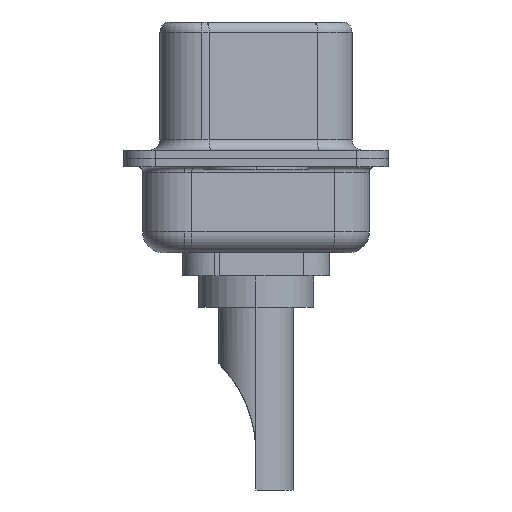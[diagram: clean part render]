
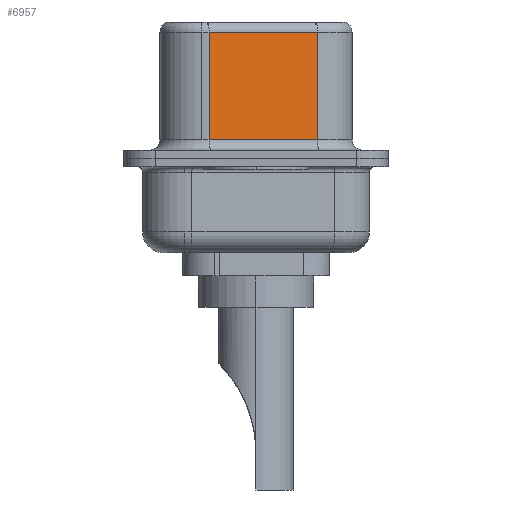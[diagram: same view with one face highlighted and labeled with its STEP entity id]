
A CAD part, left-side view. The second image highlights one B-rep face of the part: STEP entity #6957.
In plain terms, the highlighted planar face has unit normal (-0.985, -0.174, 0).
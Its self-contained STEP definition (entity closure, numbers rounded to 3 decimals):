
#53 = DIRECTION ( 'NONE',  ( -0.174, 0.985, 0. ) ) ;
#295 = ORIENTED_EDGE ( 'NONE', *, *, #6618, .T. ) ;
#870 = VECTOR ( 'NONE', #53, 1000. ) ;
#965 = EDGE_LOOP ( 'NONE', ( #12401, #5274, #295, #13449 ) ) ;
#2499 = DIRECTION ( 'NONE',  ( 0.985, 0.174, 0. ) ) ;
#2559 = CARTESIAN_POINT ( 'NONE',  ( 4.58, -2.927, 0.9 ) ) ;
#2698 = DIRECTION ( 'NONE',  ( 0.174, -0.985, 0. ) ) ;
#2806 = LINE ( 'NONE', #12154, #4554 ) ;
#3654 = LINE ( 'NONE', #13405, #870 ) ;
#4087 = AXIS2_PLACEMENT_3D ( 'NONE', #7113, #2499, #13727 ) ;
#4237 = CARTESIAN_POINT ( 'NONE',  ( 4.58, -2.927, 0.9 ) ) ;
#4554 = VECTOR ( 'NONE', #14371, 1000. ) ;
#5274 = ORIENTED_EDGE ( 'NONE', *, *, #7199, .T. ) ;
#5298 = VERTEX_POINT ( 'NONE', #12164 ) ;
#6618 = EDGE_CURVE ( 'NONE', #5298, #6783, #2806, .T. ) ;
#6783 = VERTEX_POINT ( 'NONE', #10796 ) ;
#6957 = ADVANCED_FACE ( 'NONE', ( #10961 ), #8876, .F. ) ;
#7016 = CARTESIAN_POINT ( 'NONE',  ( 4.58, -2.927, 6.52 ) ) ;
#7113 = CARTESIAN_POINT ( 'NONE',  ( 4.58, -2.927, 6.52 ) ) ;
#7149 = LINE ( 'NONE', #7016, #14067 ) ;
#7199 = EDGE_CURVE ( 'NONE', #8334, #5298, #3654, .T. ) ;
#7519 = EDGE_CURVE ( 'NONE', #8334, #12394, #7149, .T. ) ;
#8334 = VERTEX_POINT ( 'NONE', #12687 ) ;
#8876 = PLANE ( 'NONE',  #4087 ) ;
#10285 = DIRECTION ( 'NONE',  ( 0., 0., -1. ) ) ;
#10796 = CARTESIAN_POINT ( 'NONE',  ( 3.67, 2.233, 0.9 ) ) ;
#10961 = FACE_OUTER_BOUND ( 'NONE', #965, .T. ) ;
#11134 = LINE ( 'NONE', #2559, #11493 ) ;
#11493 = VECTOR ( 'NONE', #2698, 1000. ) ;
#12120 = EDGE_CURVE ( 'NONE', #6783, #12394, #11134, .T. ) ;
#12154 = CARTESIAN_POINT ( 'NONE',  ( 3.67, 2.233, 6.52 ) ) ;
#12164 = CARTESIAN_POINT ( 'NONE',  ( 3.67, 2.233, 6.02 ) ) ;
#12394 = VERTEX_POINT ( 'NONE', #4237 ) ;
#12401 = ORIENTED_EDGE ( 'NONE', *, *, #7519, .F. ) ;
#12687 = CARTESIAN_POINT ( 'NONE',  ( 4.58, -2.927, 6.02 ) ) ;
#13405 = CARTESIAN_POINT ( 'NONE',  ( 4.58, -2.927, 6.02 ) ) ;
#13449 = ORIENTED_EDGE ( 'NONE', *, *, #12120, .T. ) ;
#13727 = DIRECTION ( 'NONE',  ( -0.174, 0.985, 0. ) ) ;
#14067 = VECTOR ( 'NONE', #10285, 1000. ) ;
#14371 = DIRECTION ( 'NONE',  ( 0., 0., -1. ) ) ;
